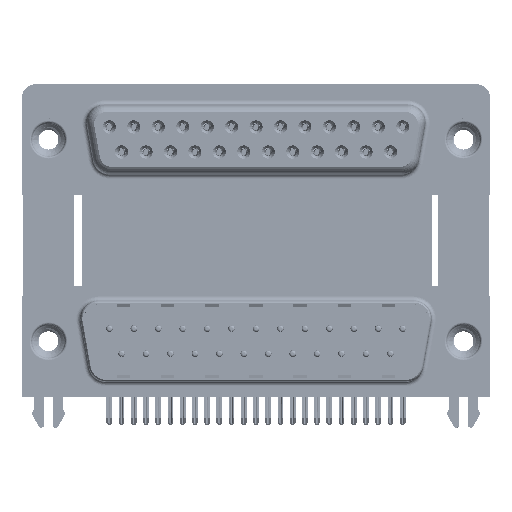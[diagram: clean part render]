
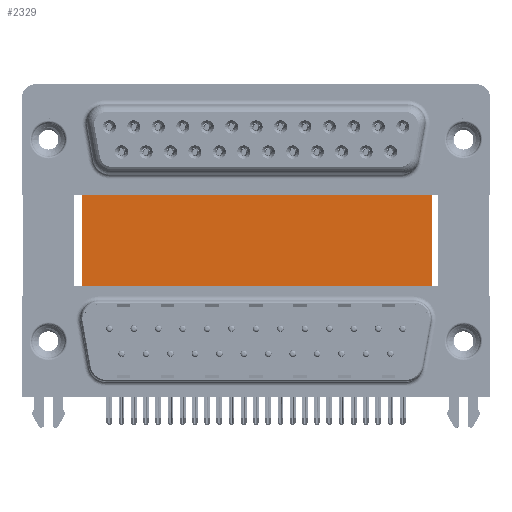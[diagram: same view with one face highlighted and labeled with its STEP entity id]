
A CAD part, top view. The second image highlights one B-rep face of the part: STEP entity #2329.
In plain terms, the highlighted planar face has unit normal (0, 0, 1).
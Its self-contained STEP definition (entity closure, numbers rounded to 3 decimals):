
#2329 = ADVANCED_FACE ( 'NONE', ( #16938 ), #43332, .F. ) ;
#3189 = LINE ( 'NONE', #56284, #17147 ) ;
#3423 = ORIENTED_EDGE ( 'NONE', *, *, #52311, .F. ) ;
#3997 = CARTESIAN_POINT ( 'NONE',  ( 3.79, 16.585, -12. ) ) ;
#7090 = CARTESIAN_POINT ( 'NONE',  ( 3.79, 16.585, -12. ) ) ;
#7465 = EDGE_CURVE ( 'NONE', #46814, #28354, #9515, .T. ) ;
#9067 = VERTEX_POINT ( 'NONE', #19905 ) ;
#9369 = AXIS2_PLACEMENT_3D ( 'NONE', #3997, #56508, #37886 ) ;
#9515 = LINE ( 'NONE', #7090, #34885 ) ;
#15098 = ORIENTED_EDGE ( 'NONE', *, *, #22360, .T. ) ;
#16257 = CARTESIAN_POINT ( 'NONE',  ( 3.79, 16.585, -12. ) ) ;
#16938 = FACE_OUTER_BOUND ( 'NONE', #23702, .T. ) ;
#17147 = VECTOR ( 'NONE', #34209, 1000. ) ;
#18313 = VECTOR ( 'NONE', #37781, 1000. ) ;
#19905 = CARTESIAN_POINT ( 'NONE',  ( 43.43, 16.585, -12. ) ) ;
#20300 = DIRECTION ( 'NONE',  ( 0., -1., 0. ) ) ;
#22360 = EDGE_CURVE ( 'NONE', #28354, #33792, #3189, .T. ) ;
#23702 = EDGE_LOOP ( 'NONE', ( #15098, #3423, #52830, #46106 ) ) ;
#24767 = CARTESIAN_POINT ( 'NONE',  ( 3.79, 16.585, -12. ) ) ;
#25082 = LINE ( 'NONE', #50898, #32376 ) ;
#26908 = CARTESIAN_POINT ( 'NONE',  ( 43.43, -3.735, -12. ) ) ;
#28354 = VERTEX_POINT ( 'NONE', #44221 ) ;
#29033 = EDGE_CURVE ( 'NONE', #46814, #9067, #38353, .T. ) ;
#32376 = VECTOR ( 'NONE', #47168, 1000. ) ;
#33792 = VERTEX_POINT ( 'NONE', #26908 ) ;
#34209 = DIRECTION ( 'NONE',  ( 1., 0., 0. ) ) ;
#34885 = VECTOR ( 'NONE', #20300, 1000. ) ;
#37781 = DIRECTION ( 'NONE',  ( 1., 0., 0. ) ) ;
#37886 = DIRECTION ( 'NONE',  ( -1., 0., 0. ) ) ;
#38353 = LINE ( 'NONE', #16257, #18313 ) ;
#43332 = PLANE ( 'NONE',  #9369 ) ;
#44221 = CARTESIAN_POINT ( 'NONE',  ( 3.79, -3.735, -12. ) ) ;
#46106 = ORIENTED_EDGE ( 'NONE', *, *, #7465, .T. ) ;
#46814 = VERTEX_POINT ( 'NONE', #24767 ) ;
#47168 = DIRECTION ( 'NONE',  ( 0., -1., 0. ) ) ;
#50898 = CARTESIAN_POINT ( 'NONE',  ( 43.43, 16.585, -12. ) ) ;
#52311 = EDGE_CURVE ( 'NONE', #9067, #33792, #25082, .T. ) ;
#52830 = ORIENTED_EDGE ( 'NONE', *, *, #29033, .F. ) ;
#56284 = CARTESIAN_POINT ( 'NONE',  ( 3.79, -3.735, -12. ) ) ;
#56508 = DIRECTION ( 'NONE',  ( 0., 0., -1. ) ) ;
